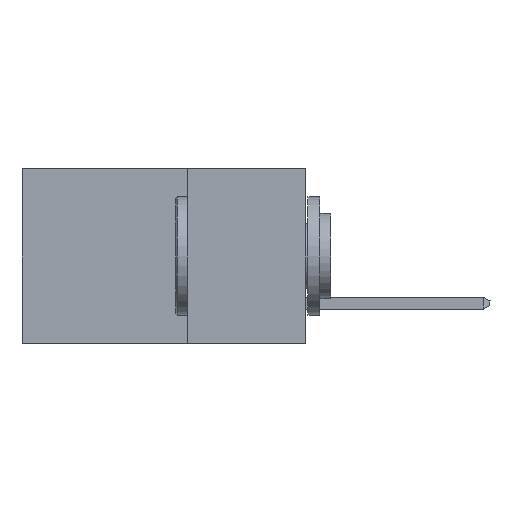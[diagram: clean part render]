
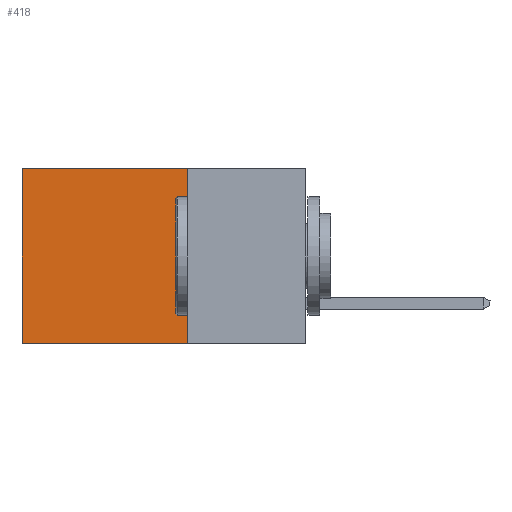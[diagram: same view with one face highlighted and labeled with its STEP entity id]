
A CAD part, left-side view. The second image highlights one B-rep face of the part: STEP entity #418.
In plain terms, the highlighted planar face has unit normal (-1, 0, 0).
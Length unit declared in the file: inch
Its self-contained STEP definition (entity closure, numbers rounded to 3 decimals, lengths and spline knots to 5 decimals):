
#418 = ADVANCED_FACE ( 'NONE', ( #4091 ), #10448, .F. ) ;
#698 = ORIENTED_EDGE ( 'NONE', *, *, #2734, .F. ) ;
#1675 = EDGE_CURVE ( 'NONE', #12463, #8443, #5650, .T. ) ;
#1881 = CARTESIAN_POINT ( 'NONE',  ( 0.2615, 0.25, -0.37 ) ) ;
#2052 = EDGE_CURVE ( 'NONE', #8443, #8502, #10014, .T. ) ;
#2559 = DIRECTION ( 'NONE',  ( 0., 1., 0. ) ) ;
#2734 = EDGE_CURVE ( 'NONE', #8933, #8502, #11457, .T. ) ;
#3112 = DIRECTION ( 'NONE',  ( 0., 0., -1. ) ) ;
#3884 = VECTOR ( 'NONE', #2559, 39.37008 ) ;
#4091 = FACE_OUTER_BOUND ( 'NONE', #13261, .T. ) ;
#4603 = CARTESIAN_POINT ( 'NONE',  ( 0.2615, 0.25, 0. ) ) ;
#4950 = CARTESIAN_POINT ( 'NONE',  ( 0.2615, 0.25, -0.37 ) ) ;
#5358 = LINE ( 'NONE', #12626, #10403 ) ;
#5477 = VECTOR ( 'NONE', #10417, 39.37008 ) ;
#5579 = ORIENTED_EDGE ( 'NONE', *, *, #2052, .T. ) ;
#5650 = LINE ( 'NONE', #4603, #3884 ) ;
#6289 = ORIENTED_EDGE ( 'NONE', *, *, #13245, .F. ) ;
#6326 = DIRECTION ( 'NONE',  ( 0., 0., -1. ) ) ;
#8443 = VERTEX_POINT ( 'NONE', #8946 ) ;
#8502 = VERTEX_POINT ( 'NONE', #12515 ) ;
#8933 = VERTEX_POINT ( 'NONE', #4950 ) ;
#8946 = CARTESIAN_POINT ( 'NONE',  ( 0.2615, 0.6, 0. ) ) ;
#8968 = CARTESIAN_POINT ( 'NONE',  ( 0.2615, 0.6, -0.37 ) ) ;
#9254 = AXIS2_PLACEMENT_3D ( 'NONE', #9609, #10370, #3112 ) ;
#9609 = CARTESIAN_POINT ( 'NONE',  ( 0.2615, 0.25, -0.37 ) ) ;
#10014 = LINE ( 'NONE', #8968, #12828 ) ;
#10370 = DIRECTION ( 'NONE',  ( 1., 0., 0. ) ) ;
#10403 = VECTOR ( 'NONE', #6326, 39.37008 ) ;
#10417 = DIRECTION ( 'NONE',  ( 0., 1., 0. ) ) ;
#10448 = PLANE ( 'NONE',  #9254 ) ;
#11198 = DIRECTION ( 'NONE',  ( 0., 0., -1. ) ) ;
#11457 = LINE ( 'NONE', #1881, #5477 ) ;
#12017 = CARTESIAN_POINT ( 'NONE',  ( 0.2615, 0.25, 0. ) ) ;
#12463 = VERTEX_POINT ( 'NONE', #12017 ) ;
#12515 = CARTESIAN_POINT ( 'NONE',  ( 0.2615, 0.6, -0.37 ) ) ;
#12626 = CARTESIAN_POINT ( 'NONE',  ( 0.2615, 0.25, -0.37 ) ) ;
#12828 = VECTOR ( 'NONE', #11198, 39.37008 ) ;
#13179 = ORIENTED_EDGE ( 'NONE', *, *, #1675, .T. ) ;
#13245 = EDGE_CURVE ( 'NONE', #12463, #8933, #5358, .T. ) ;
#13261 = EDGE_LOOP ( 'NONE', ( #5579, #698, #6289, #13179 ) ) ;
